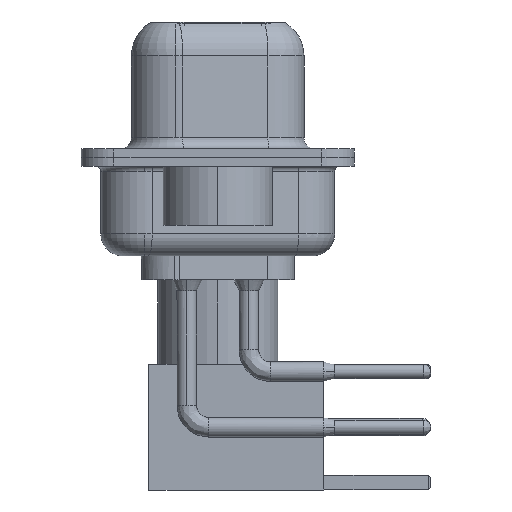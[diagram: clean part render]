
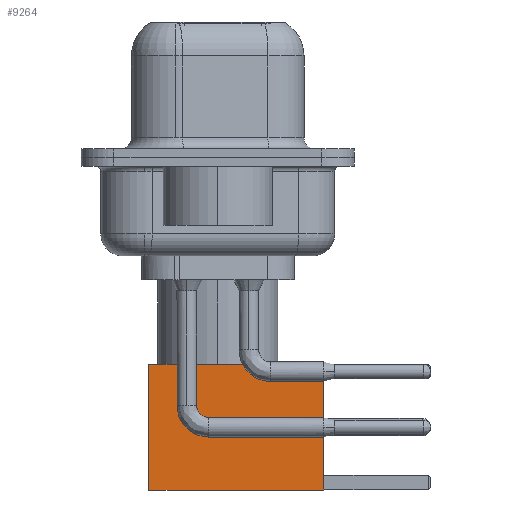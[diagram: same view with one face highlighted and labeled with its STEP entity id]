
A CAD part, left-side view. The second image highlights one B-rep face of the part: STEP entity #9264.
In plain terms, the highlighted face is planar.
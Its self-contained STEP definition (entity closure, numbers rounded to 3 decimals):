
#92 = CARTESIAN_POINT ( 'NONE',  ( 2.875, 2.875, 0. ) ) ;
#207 = LINE ( 'NONE', #13548, #17667 ) ;
#962 = VERTEX_POINT ( 'NONE', #19137 ) ;
#1189 = LINE ( 'NONE', #6241, #18995 ) ;
#1506 = CARTESIAN_POINT ( 'NONE',  ( -2.875, 2.875, 8. ) ) ;
#3756 = EDGE_CURVE ( 'NONE', #962, #17766, #4596, .T. ) ;
#4596 = LINE ( 'NONE', #11347, #10453 ) ;
#4795 = AXIS2_PLACEMENT_3D ( 'NONE', #12967, #19798, #11220 ) ;
#4928 = DIRECTION ( 'NONE',  ( 0., 0., -1. ) ) ;
#5459 = LINE ( 'NONE', #92, #20274 ) ;
#6007 = ORIENTED_EDGE ( 'NONE', *, *, #17306, .F. ) ;
#6090 = EDGE_CURVE ( 'NONE', #10779, #15951, #1189, .T. ) ;
#6241 = CARTESIAN_POINT ( 'NONE',  ( 0., 2.875, 0. ) ) ;
#6339 = PLANE ( 'NONE',  #4795 ) ;
#6469 = ORIENTED_EDGE ( 'NONE', *, *, #8908, .T. ) ;
#7080 = CARTESIAN_POINT ( 'NONE',  ( 2.875, 2.875, 0. ) ) ;
#7694 = ORIENTED_EDGE ( 'NONE', *, *, #3756, .F. ) ;
#8908 = EDGE_CURVE ( 'NONE', #962, #10779, #5459, .T. ) ;
#9264 = ADVANCED_FACE ( 'NONE', ( #9862 ), #6339, .T. ) ;
#9862 = FACE_OUTER_BOUND ( 'NONE', #12250, .T. ) ;
#10453 = VECTOR ( 'NONE', #18044, 1000. ) ;
#10779 = VERTEX_POINT ( 'NONE', #7080 ) ;
#11220 = DIRECTION ( 'NONE',  ( 0., 0., 1. ) ) ;
#11347 = CARTESIAN_POINT ( 'NONE',  ( 0., 2.875, 8. ) ) ;
#12250 = EDGE_LOOP ( 'NONE', ( #6469, #17598, #6007, #7694 ) ) ;
#12967 = CARTESIAN_POINT ( 'NONE',  ( 2.875, 2.875, 0. ) ) ;
#12978 = DIRECTION ( 'NONE',  ( -1., 0., 0. ) ) ;
#13548 = CARTESIAN_POINT ( 'NONE',  ( -2.875, 2.875, 0. ) ) ;
#15951 = VERTEX_POINT ( 'NONE', #18164 ) ;
#17306 = EDGE_CURVE ( 'NONE', #17766, #15951, #207, .T. ) ;
#17598 = ORIENTED_EDGE ( 'NONE', *, *, #6090, .T. ) ;
#17667 = VECTOR ( 'NONE', #4928, 1000. ) ;
#17766 = VERTEX_POINT ( 'NONE', #1506 ) ;
#18044 = DIRECTION ( 'NONE',  ( -1., 0., 0. ) ) ;
#18164 = CARTESIAN_POINT ( 'NONE',  ( -2.875, 2.875, 0. ) ) ;
#18913 = DIRECTION ( 'NONE',  ( 0., 0., -1. ) ) ;
#18995 = VECTOR ( 'NONE', #12978, 1000. ) ;
#19137 = CARTESIAN_POINT ( 'NONE',  ( 2.875, 2.875, 8. ) ) ;
#19798 = DIRECTION ( 'NONE',  ( 0., 1., 0. ) ) ;
#20274 = VECTOR ( 'NONE', #18913, 1000. ) ;
